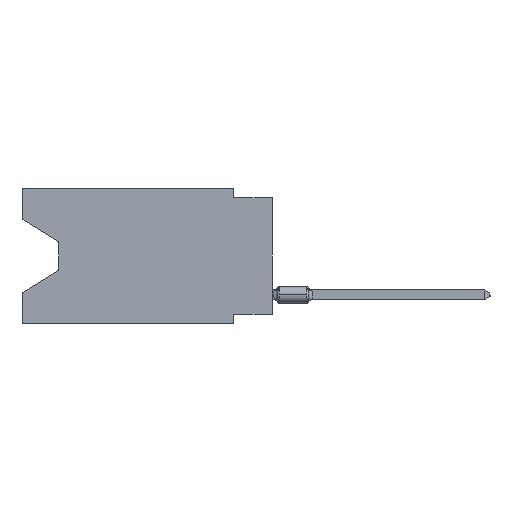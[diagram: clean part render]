
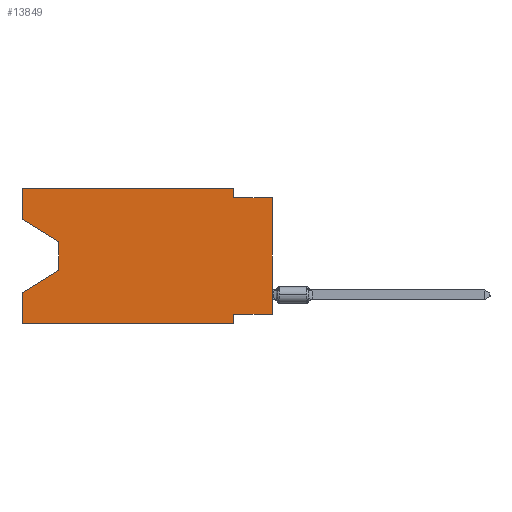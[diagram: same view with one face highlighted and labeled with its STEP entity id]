
A CAD part, left-side view. The second image highlights one B-rep face of the part: STEP entity #13849.
In plain terms, the highlighted planar face has unit normal (-1, 0, 0).
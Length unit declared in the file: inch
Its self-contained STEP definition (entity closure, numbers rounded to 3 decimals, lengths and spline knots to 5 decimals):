
#242 = CARTESIAN_POINT ( 'NONE',  ( 0., 0.1, -0.35 ) ) ;
#984 = EDGE_LOOP ( 'NONE', ( #1168, #32602, #19479, #22496, #33245, #12230, #23873, #34137, #27274, #23903, #20107, #24443 ) ) ;
#1168 = ORIENTED_EDGE ( 'NONE', *, *, #11268, .T. ) ;
#2203 = CARTESIAN_POINT ( 'NONE',  ( 0., 0.55, -0.138 ) ) ;
#3620 = VECTOR ( 'NONE', #30387, 39.37008 ) ;
#3737 = CARTESIAN_POINT ( 'NONE',  ( 0., 0., -0.325 ) ) ;
#4093 = DIRECTION ( 'NONE',  ( 0., 0., 1. ) ) ;
#4215 = EDGE_CURVE ( 'NONE', #24267, #21580, #17397, .T. ) ;
#4815 = EDGE_CURVE ( 'NONE', #26936, #4997, #9917, .T. ) ;
#4997 = VERTEX_POINT ( 'NONE', #10504 ) ;
#5451 = VERTEX_POINT ( 'NONE', #29182 ) ;
#6699 = LINE ( 'NONE', #18495, #27275 ) ;
#7000 = VECTOR ( 'NONE', #15765, 39.37008 ) ;
#7049 = CARTESIAN_POINT ( 'NONE',  ( 0., 0.645, 0. ) ) ;
#7897 = DIRECTION ( 'NONE',  ( 0., -1., 0. ) ) ;
#8286 = DIRECTION ( 'NONE',  ( 0., -0.855, -0.519 ) ) ;
#9319 = DIRECTION ( 'NONE',  ( 0., -1., 0. ) ) ;
#9718 = LINE ( 'NONE', #21521, #3620 ) ;
#9802 = VECTOR ( 'NONE', #12398, 39.37008 ) ;
#9917 = LINE ( 'NONE', #3737, #12550 ) ;
#10352 = VECTOR ( 'NONE', #9319, 39.37008 ) ;
#10504 = CARTESIAN_POINT ( 'NONE',  ( 0., 0.1, -0.325 ) ) ;
#10890 = VECTOR ( 'NONE', #4093, 39.37008 ) ;
#11010 = EDGE_CURVE ( 'NONE', #18952, #30478, #31112, .T. ) ;
#11268 = EDGE_CURVE ( 'NONE', #18952, #20285, #34972, .T. ) ;
#11784 = PLANE ( 'NONE',  #12276 ) ;
#12230 = ORIENTED_EDGE ( 'NONE', *, *, #35478, .F. ) ;
#12276 = AXIS2_PLACEMENT_3D ( 'NONE', #20673, #32466, #16983 ) ;
#12398 = DIRECTION ( 'NONE',  ( 0., 0., -1. ) ) ;
#12550 = VECTOR ( 'NONE', #18449, 39.37008 ) ;
#12715 = VECTOR ( 'NONE', #8286, 39.37008 ) ;
#12955 = EDGE_CURVE ( 'NONE', #30478, #34367, #24202, .T. ) ;
#13288 = CARTESIAN_POINT ( 'NONE',  ( 0., 0., -0.025 ) ) ;
#13849 = ADVANCED_FACE ( 'NONE', ( #20485 ), #11784, .F. ) ;
#13900 = DIRECTION ( 'NONE',  ( 0., 0., 1. ) ) ;
#13948 = VECTOR ( 'NONE', #13900, 39.37008 ) ;
#14543 = VECTOR ( 'NONE', #14821, 39.37008 ) ;
#14821 = DIRECTION ( 'NONE',  ( 0., 0.855, -0.519 ) ) ;
#15485 = EDGE_CURVE ( 'NONE', #26947, #30957, #20039, .T. ) ;
#15765 = DIRECTION ( 'NONE',  ( 0., 0., 1. ) ) ;
#16117 = CARTESIAN_POINT ( 'NONE',  ( 0., 0.645, 0. ) ) ;
#16598 = CARTESIAN_POINT ( 'NONE',  ( 0., 0., -0.025 ) ) ;
#16983 = DIRECTION ( 'NONE',  ( 0., 0., -1. ) ) ;
#17237 = CARTESIAN_POINT ( 'NONE',  ( 0., 0.645, -0.26975 ) ) ;
#17397 = LINE ( 'NONE', #32276, #23783 ) ;
#17588 = DIRECTION ( 'NONE',  ( 0., -1., 0. ) ) ;
#17759 = CARTESIAN_POINT ( 'NONE',  ( 0., 0.645, -0.08025 ) ) ;
#18449 = DIRECTION ( 'NONE',  ( 0., 1., 0. ) ) ;
#18495 = CARTESIAN_POINT ( 'NONE',  ( 0., 0.1, 0. ) ) ;
#18660 = CARTESIAN_POINT ( 'NONE',  ( 0., 0., -0.325 ) ) ;
#18715 = LINE ( 'NONE', #16598, #21041 ) ;
#18952 = VERTEX_POINT ( 'NONE', #17759 ) ;
#19479 = ORIENTED_EDGE ( 'NONE', *, *, #15485, .T. ) ;
#19910 = CARTESIAN_POINT ( 'NONE',  ( 0., 0.645, 0. ) ) ;
#20039 = LINE ( 'NONE', #31622, #14543 ) ;
#20107 = ORIENTED_EDGE ( 'NONE', *, *, #12955, .F. ) ;
#20285 = VERTEX_POINT ( 'NONE', #2203 ) ;
#20485 = FACE_OUTER_BOUND ( 'NONE', #984, .T. ) ;
#20673 = CARTESIAN_POINT ( 'NONE',  ( 0., 0.645, 0. ) ) ;
#21041 = VECTOR ( 'NONE', #7897, 39.37008 ) ;
#21472 = CARTESIAN_POINT ( 'NONE',  ( 0., 0.645, 0. ) ) ;
#21521 = CARTESIAN_POINT ( 'NONE',  ( 0., 0.1, -0.35 ) ) ;
#21580 = VERTEX_POINT ( 'NONE', #242 ) ;
#21698 = CARTESIAN_POINT ( 'NONE',  ( 0., 0., 0. ) ) ;
#21862 = CARTESIAN_POINT ( 'NONE',  ( 0., 0.645, -0.35 ) ) ;
#22496 = ORIENTED_EDGE ( 'NONE', *, *, #27053, .F. ) ;
#23634 = EDGE_CURVE ( 'NONE', #5451, #37109, #18715, .T. ) ;
#23783 = VECTOR ( 'NONE', #17588, 39.37008 ) ;
#23873 = ORIENTED_EDGE ( 'NONE', *, *, #4815, .F. ) ;
#23903 = ORIENTED_EDGE ( 'NONE', *, *, #25085, .F. ) ;
#24024 = CARTESIAN_POINT ( 'NONE',  ( 0., 0.55, -0.138 ) ) ;
#24202 = LINE ( 'NONE', #21472, #10352 ) ;
#24267 = VERTEX_POINT ( 'NONE', #21862 ) ;
#24443 = ORIENTED_EDGE ( 'NONE', *, *, #11010, .F. ) ;
#24487 = DIRECTION ( 'NONE',  ( 0., 0., -1. ) ) ;
#25085 = EDGE_CURVE ( 'NONE', #34367, #5451, #6699, .T. ) ;
#26270 = CARTESIAN_POINT ( 'NONE',  ( 0., 0.1, 0. ) ) ;
#26645 = CARTESIAN_POINT ( 'NONE',  ( 0., 0.55, -0.212 ) ) ;
#26936 = VERTEX_POINT ( 'NONE', #18660 ) ;
#26947 = VERTEX_POINT ( 'NONE', #26645 ) ;
#27053 = EDGE_CURVE ( 'NONE', #24267, #30957, #30652, .T. ) ;
#27274 = ORIENTED_EDGE ( 'NONE', *, *, #23634, .F. ) ;
#27275 = VECTOR ( 'NONE', #24487, 39.37008 ) ;
#27693 = LINE ( 'NONE', #21698, #10890 ) ;
#29182 = CARTESIAN_POINT ( 'NONE',  ( 0., 0.1, -0.025 ) ) ;
#29595 = EDGE_CURVE ( 'NONE', #26936, #37109, #27693, .T. ) ;
#30387 = DIRECTION ( 'NONE',  ( 0., 0., -1. ) ) ;
#30478 = VERTEX_POINT ( 'NONE', #16117 ) ;
#30524 = LINE ( 'NONE', #24024, #9802 ) ;
#30652 = LINE ( 'NONE', #7049, #7000 ) ;
#30957 = VERTEX_POINT ( 'NONE', #17237 ) ;
#31112 = LINE ( 'NONE', #19910, #13948 ) ;
#31622 = CARTESIAN_POINT ( 'NONE',  ( 0., 0.55, -0.212 ) ) ;
#32276 = CARTESIAN_POINT ( 'NONE',  ( 0., 0.645, -0.35 ) ) ;
#32466 = DIRECTION ( 'NONE',  ( 1., 0., 0. ) ) ;
#32602 = ORIENTED_EDGE ( 'NONE', *, *, #35872, .T. ) ;
#33245 = ORIENTED_EDGE ( 'NONE', *, *, #4215, .T. ) ;
#34137 = ORIENTED_EDGE ( 'NONE', *, *, #29595, .T. ) ;
#34367 = VERTEX_POINT ( 'NONE', #26270 ) ;
#34769 = CARTESIAN_POINT ( 'NONE',  ( 0., 0.645, -0.08025 ) ) ;
#34972 = LINE ( 'NONE', #34769, #12715 ) ;
#35478 = EDGE_CURVE ( 'NONE', #4997, #21580, #9718, .T. ) ;
#35872 = EDGE_CURVE ( 'NONE', #20285, #26947, #30524, .T. ) ;
#37109 = VERTEX_POINT ( 'NONE', #13288 ) ;
